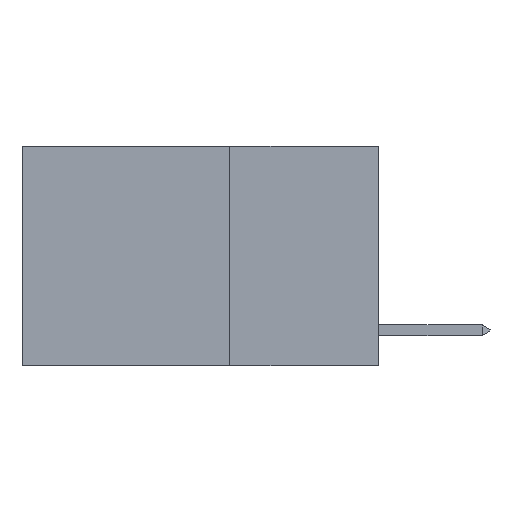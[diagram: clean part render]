
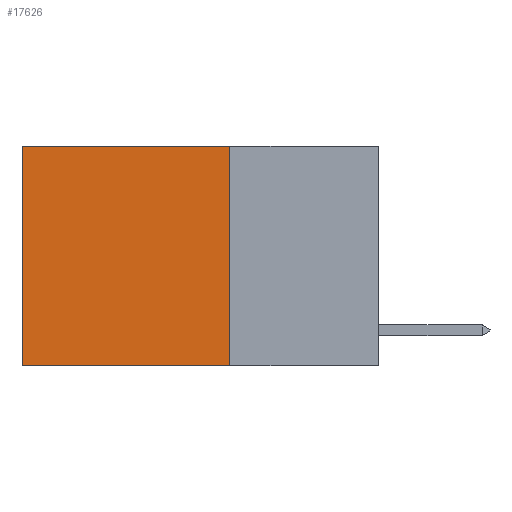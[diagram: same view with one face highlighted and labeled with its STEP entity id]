
A CAD part, left-side view. The second image highlights one B-rep face of the part: STEP entity #17626.
In plain terms, the highlighted planar face has unit normal (-1, 0, 0).
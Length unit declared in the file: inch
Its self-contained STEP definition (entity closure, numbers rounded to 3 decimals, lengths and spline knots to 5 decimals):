
#694 = LINE ( 'NONE', #9446, #16402 ) ;
#1641 = DIRECTION ( 'NONE',  ( 0., 0., -1. ) ) ;
#1885 = CARTESIAN_POINT ( 'NONE',  ( 0.2625, 0.25, 0. ) ) ;
#1993 = AXIS2_PLACEMENT_3D ( 'NONE', #1885, #2175, #28446 ) ;
#2138 = VERTEX_POINT ( 'NONE', #21266 ) ;
#2175 = DIRECTION ( 'NONE',  ( 1., 0., 0. ) ) ;
#2877 = LINE ( 'NONE', #23319, #7464 ) ;
#3025 = VECTOR ( 'NONE', #11890, 39.37008 ) ;
#3865 = ORIENTED_EDGE ( 'NONE', *, *, #16474, .F. ) ;
#7464 = VECTOR ( 'NONE', #23459, 39.37008 ) ;
#7612 = CARTESIAN_POINT ( 'NONE',  ( 0.2625, 0.25, 0. ) ) ;
#7870 = VERTEX_POINT ( 'NONE', #14677 ) ;
#8173 = EDGE_CURVE ( 'NONE', #7870, #18896, #9666, .T. ) ;
#9291 = DIRECTION ( 'NONE',  ( 0., 1., 0. ) ) ;
#9446 = CARTESIAN_POINT ( 'NONE',  ( 0.2625, 0.25, -0.37 ) ) ;
#9505 = ORIENTED_EDGE ( 'NONE', *, *, #8173, .T. ) ;
#9666 = LINE ( 'NONE', #7612, #3025 ) ;
#10687 = ORIENTED_EDGE ( 'NONE', *, *, #15599, .F. ) ;
#11890 = DIRECTION ( 'NONE',  ( 0., 1., 0. ) ) ;
#14076 = CARTESIAN_POINT ( 'NONE',  ( 0.2625, 0.6, 0. ) ) ;
#14152 = EDGE_LOOP ( 'NONE', ( #22233, #3865, #10687, #9505 ) ) ;
#14677 = CARTESIAN_POINT ( 'NONE',  ( 0.2625, 0.25, 0. ) ) ;
#14969 = VECTOR ( 'NONE', #1641, 39.37008 ) ;
#15599 = EDGE_CURVE ( 'NONE', #7870, #23949, #21784, .T. ) ;
#16402 = VECTOR ( 'NONE', #9291, 39.37008 ) ;
#16474 = EDGE_CURVE ( 'NONE', #23949, #2138, #694, .T. ) ;
#17626 = ADVANCED_FACE ( 'NONE', ( #22323 ), #26695, .F. ) ;
#18896 = VERTEX_POINT ( 'NONE', #14076 ) ;
#21266 = CARTESIAN_POINT ( 'NONE',  ( 0.2625, 0.6, -0.37 ) ) ;
#21784 = LINE ( 'NONE', #24113, #14969 ) ;
#22233 = ORIENTED_EDGE ( 'NONE', *, *, #22731, .T. ) ;
#22323 = FACE_OUTER_BOUND ( 'NONE', #14152, .T. ) ;
#22731 = EDGE_CURVE ( 'NONE', #18896, #2138, #2877, .T. ) ;
#23319 = CARTESIAN_POINT ( 'NONE',  ( 0.2625, 0.6, 0. ) ) ;
#23459 = DIRECTION ( 'NONE',  ( 0., 0., -1. ) ) ;
#23949 = VERTEX_POINT ( 'NONE', #28632 ) ;
#24113 = CARTESIAN_POINT ( 'NONE',  ( 0.2625, 0.25, 0. ) ) ;
#26695 = PLANE ( 'NONE',  #1993 ) ;
#28446 = DIRECTION ( 'NONE',  ( 0., 0., -1. ) ) ;
#28632 = CARTESIAN_POINT ( 'NONE',  ( 0.2625, 0.25, -0.37 ) ) ;
